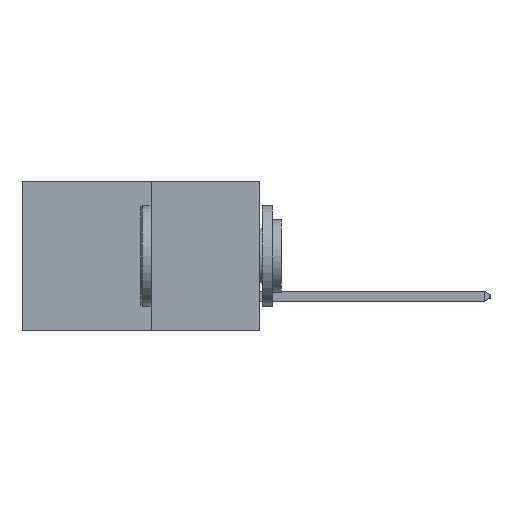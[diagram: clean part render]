
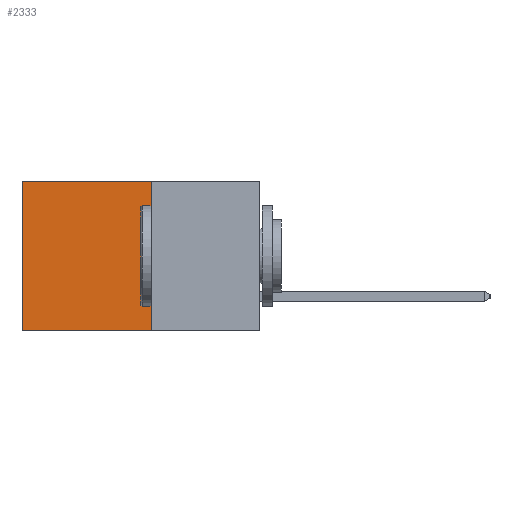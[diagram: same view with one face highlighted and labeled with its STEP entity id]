
A CAD part, left-side view. The second image highlights one B-rep face of the part: STEP entity #2333.
In plain terms, the highlighted planar face has unit normal (-1, 0, 0).
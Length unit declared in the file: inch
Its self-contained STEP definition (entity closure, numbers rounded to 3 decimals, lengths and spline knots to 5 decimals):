
#122 = LINE ( 'NONE', #10189, #11032 ) ;
#689 = EDGE_LOOP ( 'NONE', ( #6723, #26422, #18793, #16347 ) ) ;
#814 = CARTESIAN_POINT ( 'NONE',  ( 0.277, 0.59, -0.37 ) ) ;
#2333 = ADVANCED_FACE ( 'NONE', ( #18138 ), #26624, .F. ) ;
#2822 = VERTEX_POINT ( 'NONE', #25176 ) ;
#2992 = DIRECTION ( 'NONE',  ( 0., 0., -1. ) ) ;
#3141 = CARTESIAN_POINT ( 'NONE',  ( 0.277, 0.27, 0. ) ) ;
#3432 = CARTESIAN_POINT ( 'NONE',  ( 0.277, 0.59, -0.37 ) ) ;
#4065 = VECTOR ( 'NONE', #16136, 39.37008 ) ;
#5377 = CARTESIAN_POINT ( 'NONE',  ( 0.277, 0.27, -0.37 ) ) ;
#6538 = VECTOR ( 'NONE', #18241, 39.37008 ) ;
#6723 = ORIENTED_EDGE ( 'NONE', *, *, #21629, .T. ) ;
#9203 = VECTOR ( 'NONE', #2992, 39.37008 ) ;
#9885 = EDGE_CURVE ( 'NONE', #18852, #12201, #122, .T. ) ;
#10189 = CARTESIAN_POINT ( 'NONE',  ( 0.277, 0.27, -0.37 ) ) ;
#11032 = VECTOR ( 'NONE', #16628, 39.37008 ) ;
#11674 = LINE ( 'NONE', #3141, #6538 ) ;
#12081 = EDGE_CURVE ( 'NONE', #15773, #18852, #21244, .T. ) ;
#12201 = VERTEX_POINT ( 'NONE', #3432 ) ;
#13847 = CARTESIAN_POINT ( 'NONE',  ( 0.277, 0.27, 0. ) ) ;
#15401 = CARTESIAN_POINT ( 'NONE',  ( 0.277, 0.27, -0.37 ) ) ;
#15773 = VERTEX_POINT ( 'NONE', #13847 ) ;
#16136 = DIRECTION ( 'NONE',  ( 0., 0., -1. ) ) ;
#16347 = ORIENTED_EDGE ( 'NONE', *, *, #19033, .T. ) ;
#16628 = DIRECTION ( 'NONE',  ( 0., 1., 0. ) ) ;
#18138 = FACE_OUTER_BOUND ( 'NONE', #689, .T. ) ;
#18241 = DIRECTION ( 'NONE',  ( 0., 1., 0. ) ) ;
#18793 = ORIENTED_EDGE ( 'NONE', *, *, #12081, .F. ) ;
#18852 = VERTEX_POINT ( 'NONE', #15401 ) ;
#19033 = EDGE_CURVE ( 'NONE', #15773, #2822, #11674, .T. ) ;
#19039 = AXIS2_PLACEMENT_3D ( 'NONE', #26532, #26498, #26712 ) ;
#21244 = LINE ( 'NONE', #5377, #4065 ) ;
#21629 = EDGE_CURVE ( 'NONE', #2822, #12201, #26101, .T. ) ;
#25176 = CARTESIAN_POINT ( 'NONE',  ( 0.277, 0.59, 0. ) ) ;
#26101 = LINE ( 'NONE', #814, #9203 ) ;
#26422 = ORIENTED_EDGE ( 'NONE', *, *, #9885, .F. ) ;
#26498 = DIRECTION ( 'NONE',  ( 1., 0., 0. ) ) ;
#26532 = CARTESIAN_POINT ( 'NONE',  ( 0.277, 0.27, -0.37 ) ) ;
#26624 = PLANE ( 'NONE',  #19039 ) ;
#26712 = DIRECTION ( 'NONE',  ( 0., 0., -1. ) ) ;
